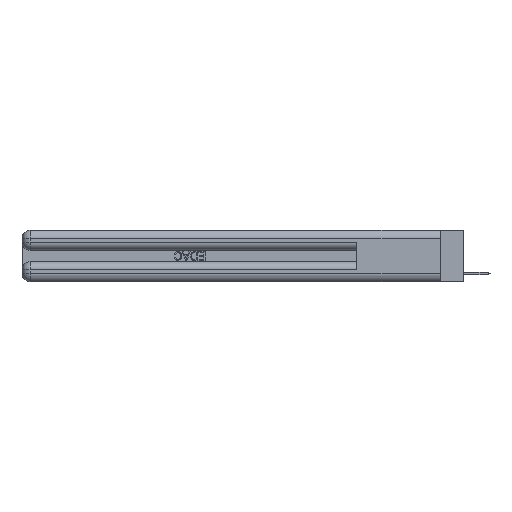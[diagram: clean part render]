
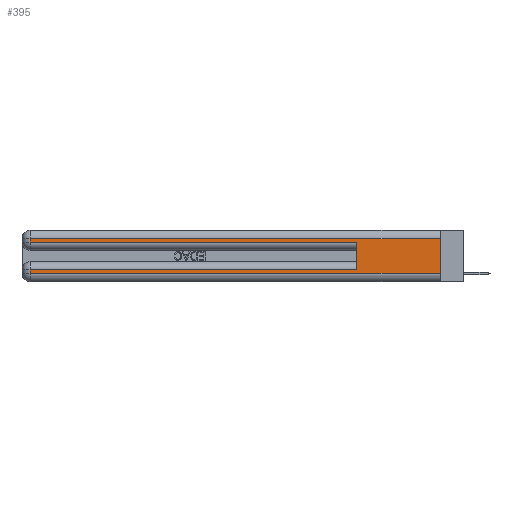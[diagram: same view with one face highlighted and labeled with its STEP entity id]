
A CAD part, left-side view. The second image highlights one B-rep face of the part: STEP entity #395.
In plain terms, the highlighted planar face has unit normal (-1, 0, 0).
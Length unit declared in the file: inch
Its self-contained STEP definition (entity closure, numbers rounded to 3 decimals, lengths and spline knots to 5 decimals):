
#104 = ORIENTED_EDGE ( 'NONE', *, *, #12753, .T. ) ;
#395 = ADVANCED_FACE ( 'NONE', ( #5089 ), #1345, .F. ) ;
#616 = CARTESIAN_POINT ( 'NONE',  ( 0., 0., 0.31 ) ) ;
#650 = CARTESIAN_POINT ( 'NONE',  ( 0., 2.94, 0.37 ) ) ;
#1290 = CARTESIAN_POINT ( 'NONE',  ( 0., 2.94, 0.085 ) ) ;
#1345 = PLANE ( 'NONE',  #22175 ) ;
#1647 = EDGE_CURVE ( 'NONE', #27602, #19796, #11929, .T. ) ;
#2936 = ORIENTED_EDGE ( 'NONE', *, *, #24838, .T. ) ;
#3133 = ORIENTED_EDGE ( 'NONE', *, *, #10244, .F. ) ;
#3220 = LINE ( 'NONE', #17656, #16812 ) ;
#3597 = VECTOR ( 'NONE', #18975, 39.37008 ) ;
#4145 = VECTOR ( 'NONE', #25527, 39.37008 ) ;
#5089 = FACE_OUTER_BOUND ( 'NONE', #15662, .T. ) ;
#5710 = ORIENTED_EDGE ( 'NONE', *, *, #24635, .T. ) ;
#6920 = EDGE_CURVE ( 'NONE', #8417, #24658, #21136, .T. ) ;
#8005 = VECTOR ( 'NONE', #9637, 39.37008 ) ;
#8221 = CARTESIAN_POINT ( 'NONE',  ( 0., 0., 0.06 ) ) ;
#8335 = CARTESIAN_POINT ( 'NONE',  ( 0., 0., 0.37 ) ) ;
#8417 = VERTEX_POINT ( 'NONE', #616 ) ;
#8515 = CARTESIAN_POINT ( 'NONE',  ( 0., 2.94, 0.06 ) ) ;
#8821 = DIRECTION ( 'NONE',  ( 0., -1., 0. ) ) ;
#9637 = DIRECTION ( 'NONE',  ( 0., 0., -1. ) ) ;
#9964 = LINE ( 'NONE', #8221, #12333 ) ;
#10244 = EDGE_CURVE ( 'NONE', #13933, #11635, #23386, .T. ) ;
#10284 = DIRECTION ( 'NONE',  ( 0., 1., 0. ) ) ;
#10550 = VECTOR ( 'NONE', #16296, 39.37008 ) ;
#10618 = ORIENTED_EDGE ( 'NONE', *, *, #6920, .F. ) ;
#11635 = VERTEX_POINT ( 'NONE', #15229 ) ;
#11844 = VECTOR ( 'NONE', #24797, 39.37008 ) ;
#11929 = LINE ( 'NONE', #20616, #10550 ) ;
#11994 = CARTESIAN_POINT ( 'NONE',  ( 0., 0.6, 0.145 ) ) ;
#12257 = DIRECTION ( 'NONE',  ( 1., 0., 0. ) ) ;
#12333 = VECTOR ( 'NONE', #27870, 39.37008 ) ;
#12753 = EDGE_CURVE ( 'NONE', #22490, #27891, #13782, .T. ) ;
#13782 = LINE ( 'NONE', #650, #8005 ) ;
#13933 = VERTEX_POINT ( 'NONE', #22445 ) ;
#14306 = ORIENTED_EDGE ( 'NONE', *, *, #1647, .T. ) ;
#15229 = CARTESIAN_POINT ( 'NONE',  ( 0., 0.6, 0.285 ) ) ;
#15662 = EDGE_LOOP ( 'NONE', ( #10618, #2936, #14306, #17836, #3133, #20832, #104, #5710 ) ) ;
#16296 = DIRECTION ( 'NONE',  ( 0., 0., -1. ) ) ;
#16404 = VECTOR ( 'NONE', #10284, 39.37008 ) ;
#16441 = CARTESIAN_POINT ( 'NONE',  ( 0., 0., 0.31 ) ) ;
#16812 = VECTOR ( 'NONE', #8821, 39.37008 ) ;
#17656 = CARTESIAN_POINT ( 'NONE',  ( 0., 0., 0.285 ) ) ;
#17836 = ORIENTED_EDGE ( 'NONE', *, *, #20085, .T. ) ;
#18798 = DIRECTION ( 'NONE',  ( 0., 0., -1. ) ) ;
#18975 = DIRECTION ( 'NONE',  ( 0., 1., 0. ) ) ;
#19796 = VERTEX_POINT ( 'NONE', #20726 ) ;
#20085 = EDGE_CURVE ( 'NONE', #19796, #11635, #3220, .T. ) ;
#20616 = CARTESIAN_POINT ( 'NONE',  ( 0., 2.94, 0.37 ) ) ;
#20726 = CARTESIAN_POINT ( 'NONE',  ( 0., 2.94, 0.285 ) ) ;
#20736 = CARTESIAN_POINT ( 'NONE',  ( 0., 2.94, 0.31 ) ) ;
#20832 = ORIENTED_EDGE ( 'NONE', *, *, #27229, .T. ) ;
#21076 = CARTESIAN_POINT ( 'NONE',  ( 0., 0., 0.085 ) ) ;
#21136 = LINE ( 'NONE', #8335, #4145 ) ;
#22175 = AXIS2_PLACEMENT_3D ( 'NONE', #25261, #12257, #18798 ) ;
#22445 = CARTESIAN_POINT ( 'NONE',  ( 0., 0.6, 0.085 ) ) ;
#22490 = VERTEX_POINT ( 'NONE', #1290 ) ;
#23386 = LINE ( 'NONE', #11994, #11844 ) ;
#23412 = CARTESIAN_POINT ( 'NONE',  ( 0., 0., 0.06 ) ) ;
#24635 = EDGE_CURVE ( 'NONE', #27891, #24658, #9964, .T. ) ;
#24658 = VERTEX_POINT ( 'NONE', #23412 ) ;
#24687 = LINE ( 'NONE', #21076, #3597 ) ;
#24797 = DIRECTION ( 'NONE',  ( 0., 0., 1. ) ) ;
#24838 = EDGE_CURVE ( 'NONE', #8417, #27602, #27952, .T. ) ;
#25261 = CARTESIAN_POINT ( 'NONE',  ( 0., 0., 0.37 ) ) ;
#25527 = DIRECTION ( 'NONE',  ( 0., 0., -1. ) ) ;
#27229 = EDGE_CURVE ( 'NONE', #13933, #22490, #24687, .T. ) ;
#27602 = VERTEX_POINT ( 'NONE', #20736 ) ;
#27870 = DIRECTION ( 'NONE',  ( 0., -1., 0. ) ) ;
#27891 = VERTEX_POINT ( 'NONE', #8515 ) ;
#27952 = LINE ( 'NONE', #16441, #16404 ) ;
